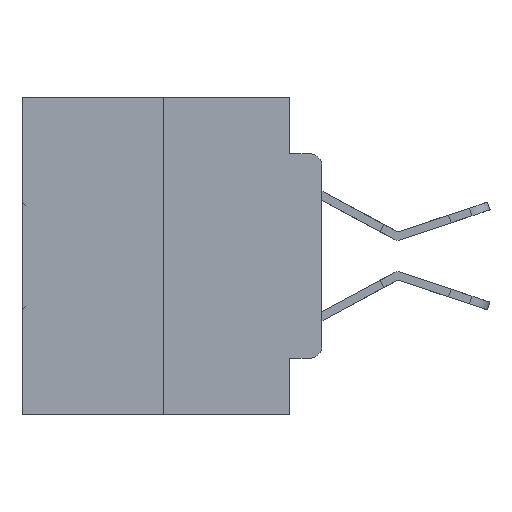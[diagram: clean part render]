
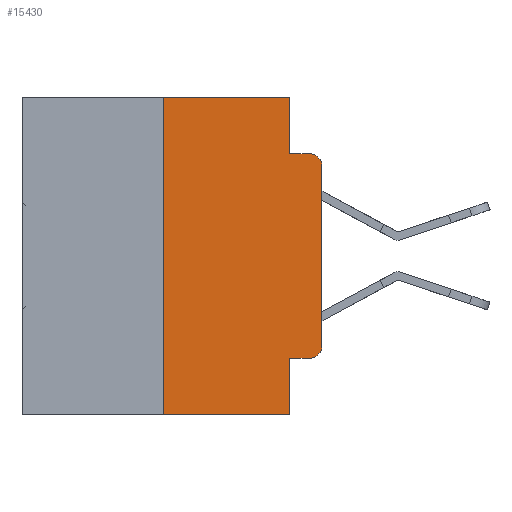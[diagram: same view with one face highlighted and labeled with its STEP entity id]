
A CAD part, left-side view. The second image highlights one B-rep face of the part: STEP entity #15430.
In plain terms, the highlighted planar face has unit normal (-1, 0, 0).
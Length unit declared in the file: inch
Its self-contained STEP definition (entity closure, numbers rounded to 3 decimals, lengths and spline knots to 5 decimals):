
#855 = DIRECTION ( 'NONE',  ( 0., -1., 0. ) ) ;
#979 = CARTESIAN_POINT ( 'NONE',  ( 0., 0.02, -0.0885 ) ) ;
#1496 = LINE ( 'NONE', #13788, #27185 ) ;
#1937 = VERTEX_POINT ( 'NONE', #7492 ) ;
#2089 = EDGE_CURVE ( 'NONE', #1937, #2124, #12134, .T. ) ;
#2124 = VERTEX_POINT ( 'NONE', #22237 ) ;
#3092 = ORIENTED_EDGE ( 'NONE', *, *, #22532, .F. ) ;
#3229 = FACE_OUTER_BOUND ( 'NONE', #13046, .T. ) ;
#3327 = CIRCLE ( 'NONE', #18204, 0.02 ) ;
#4224 = VECTOR ( 'NONE', #20639, 39.37008 ) ;
#4677 = LINE ( 'NONE', #19504, #17240 ) ;
#4921 = CARTESIAN_POINT ( 'NONE',  ( 0., 0.02, -0.1085 ) ) ;
#5753 = CARTESIAN_POINT ( 'NONE',  ( 0., 0., 0. ) ) ;
#7487 = DIRECTION ( 'NONE',  ( 0., 0., -1. ) ) ;
#7492 = CARTESIAN_POINT ( 'NONE',  ( 0., 0.051, -0.4115 ) ) ;
#7564 = EDGE_CURVE ( 'NONE', #17624, #8543, #24611, .T. ) ;
#8543 = VERTEX_POINT ( 'NONE', #979 ) ;
#8568 = EDGE_CURVE ( 'NONE', #1937, #31199, #1496, .T. ) ;
#9446 = CARTESIAN_POINT ( 'NONE',  ( 0., 0.02, -0.4115 ) ) ;
#9901 = CARTESIAN_POINT ( 'NONE',  ( 0., 0.473, 0. ) ) ;
#9990 = EDGE_CURVE ( 'NONE', #21151, #23198, #4677, .T. ) ;
#10076 = DIRECTION ( 'NONE',  ( -1., 0., 0. ) ) ;
#11289 = DIRECTION ( 'NONE',  ( 0., -1., 0. ) ) ;
#12095 = DIRECTION ( 'NONE',  ( 0., 0., -1. ) ) ;
#12134 = LINE ( 'NONE', #31703, #30045 ) ;
#12912 = CARTESIAN_POINT ( 'NONE',  ( 0., 0., -0.1085 ) ) ;
#13046 = EDGE_LOOP ( 'NONE', ( #31983, #19927, #21461, #3092, #22974, #17289, #30157, #24515, #18810, #31650 ) ) ;
#13425 = CARTESIAN_POINT ( 'NONE',  ( 0., 0.473, -0.5 ) ) ;
#13788 = CARTESIAN_POINT ( 'NONE',  ( 0., 0.051, -0.4115 ) ) ;
#14484 = EDGE_CURVE ( 'NONE', #21151, #2124, #16722, .T. ) ;
#14669 = LINE ( 'NONE', #24967, #26887 ) ;
#15430 = ADVANCED_FACE ( 'NONE', ( #3229 ), #19406, .F. ) ;
#15508 = DIRECTION ( 'NONE',  ( 0., 0., -1. ) ) ;
#15938 = DIRECTION ( 'NONE',  ( 0., -1., 0. ) ) ;
#16018 = VERTEX_POINT ( 'NONE', #16941 ) ;
#16722 = LINE ( 'NONE', #13425, #28087 ) ;
#16941 = CARTESIAN_POINT ( 'NONE',  ( 0., 0.051, 0. ) ) ;
#17240 = VECTOR ( 'NONE', #21950, 39.37008 ) ;
#17289 = ORIENTED_EDGE ( 'NONE', *, *, #9990, .F. ) ;
#17388 = VERTEX_POINT ( 'NONE', #20135 ) ;
#17424 = VERTEX_POINT ( 'NONE', #12912 ) ;
#17624 = VERTEX_POINT ( 'NONE', #25882 ) ;
#18204 = AXIS2_PLACEMENT_3D ( 'NONE', #24801, #10076, #27211 ) ;
#18519 = CIRCLE ( 'NONE', #28000, 0.02 ) ;
#18810 = ORIENTED_EDGE ( 'NONE', *, *, #8568, .T. ) ;
#19406 = PLANE ( 'NONE',  #26640 ) ;
#19504 = CARTESIAN_POINT ( 'NONE',  ( 0., 0.25, 0. ) ) ;
#19807 = EDGE_CURVE ( 'NONE', #31199, #17388, #3327, .T. ) ;
#19927 = ORIENTED_EDGE ( 'NONE', *, *, #22424, .T. ) ;
#20135 = CARTESIAN_POINT ( 'NONE',  ( 0., 0., -0.3915 ) ) ;
#20333 = CARTESIAN_POINT ( 'NONE',  ( 0., 0.25, 0. ) ) ;
#20639 = DIRECTION ( 'NONE',  ( 0., 0., 1. ) ) ;
#21151 = VERTEX_POINT ( 'NONE', #27458 ) ;
#21461 = ORIENTED_EDGE ( 'NONE', *, *, #7564, .F. ) ;
#21749 = CARTESIAN_POINT ( 'NONE',  ( 0., 0.473, 0. ) ) ;
#21950 = DIRECTION ( 'NONE',  ( 0., 0., 1. ) ) ;
#22237 = CARTESIAN_POINT ( 'NONE',  ( 0., 0.051, -0.5 ) ) ;
#22308 = DIRECTION ( 'NONE',  ( -1., 0., 0. ) ) ;
#22424 = EDGE_CURVE ( 'NONE', #17424, #8543, #18519, .T. ) ;
#22532 = EDGE_CURVE ( 'NONE', #16018, #17624, #14669, .T. ) ;
#22974 = ORIENTED_EDGE ( 'NONE', *, *, #29140, .F. ) ;
#23198 = VERTEX_POINT ( 'NONE', #20333 ) ;
#23797 = VECTOR ( 'NONE', #24628, 39.37008 ) ;
#24515 = ORIENTED_EDGE ( 'NONE', *, *, #2089, .F. ) ;
#24560 = LINE ( 'NONE', #9901, #23797 ) ;
#24611 = LINE ( 'NONE', #28161, #26153 ) ;
#24628 = DIRECTION ( 'NONE',  ( 0., -1., 0. ) ) ;
#24801 = CARTESIAN_POINT ( 'NONE',  ( 0., 0.02, -0.3915 ) ) ;
#24967 = CARTESIAN_POINT ( 'NONE',  ( 0., 0.051, 0. ) ) ;
#25662 = EDGE_CURVE ( 'NONE', #17388, #17424, #30433, .T. ) ;
#25882 = CARTESIAN_POINT ( 'NONE',  ( 0., 0.051, -0.0885 ) ) ;
#26153 = VECTOR ( 'NONE', #855, 39.37008 ) ;
#26640 = AXIS2_PLACEMENT_3D ( 'NONE', #21749, #26758, #12095 ) ;
#26758 = DIRECTION ( 'NONE',  ( 1., 0., 0. ) ) ;
#26887 = VECTOR ( 'NONE', #27380, 39.37008 ) ;
#27185 = VECTOR ( 'NONE', #11289, 39.37008 ) ;
#27211 = DIRECTION ( 'NONE',  ( 0., 0., -1. ) ) ;
#27380 = DIRECTION ( 'NONE',  ( 0., 0., -1. ) ) ;
#27458 = CARTESIAN_POINT ( 'NONE',  ( 0., 0.25, -0.5 ) ) ;
#28000 = AXIS2_PLACEMENT_3D ( 'NONE', #4921, #22308, #7487 ) ;
#28087 = VECTOR ( 'NONE', #15938, 39.37008 ) ;
#28161 = CARTESIAN_POINT ( 'NONE',  ( 0., 0.051, -0.0885 ) ) ;
#29140 = EDGE_CURVE ( 'NONE', #23198, #16018, #24560, .T. ) ;
#30045 = VECTOR ( 'NONE', #15508, 39.37008 ) ;
#30157 = ORIENTED_EDGE ( 'NONE', *, *, #14484, .T. ) ;
#30433 = LINE ( 'NONE', #5753, #4224 ) ;
#31199 = VERTEX_POINT ( 'NONE', #9446 ) ;
#31650 = ORIENTED_EDGE ( 'NONE', *, *, #19807, .T. ) ;
#31703 = CARTESIAN_POINT ( 'NONE',  ( 0., 0.051, 0. ) ) ;
#31983 = ORIENTED_EDGE ( 'NONE', *, *, #25662, .T. ) ;
